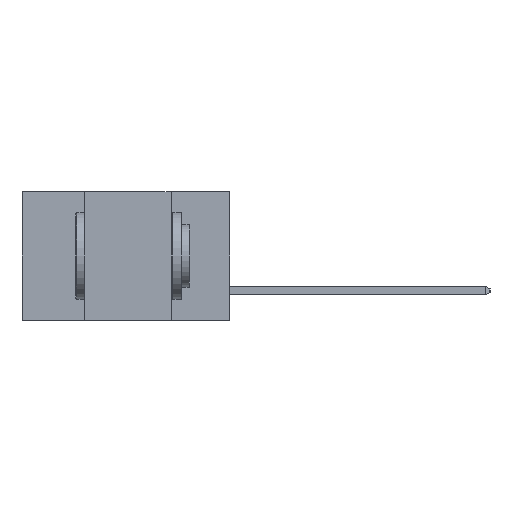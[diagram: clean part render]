
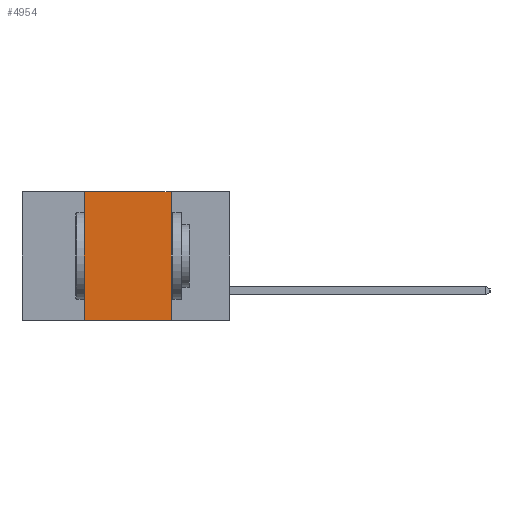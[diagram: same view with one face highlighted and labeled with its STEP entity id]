
A CAD part, left-side view. The second image highlights one B-rep face of the part: STEP entity #4954.
In plain terms, the highlighted planar face has unit normal (-1, 0, 0).
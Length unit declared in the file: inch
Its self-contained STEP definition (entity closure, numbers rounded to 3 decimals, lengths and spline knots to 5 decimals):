
#1108 = LINE ( 'NONE', #4610, #4669 ) ;
#2215 = LINE ( 'NONE', #11364, #16387 ) ;
#2260 = CARTESIAN_POINT ( 'NONE',  ( 0., 0.6, -0.37 ) ) ;
#2921 = CARTESIAN_POINT ( 'NONE',  ( 0., 0.42, 0. ) ) ;
#3185 = EDGE_CURVE ( 'NONE', #5543, #7840, #6414, .T. ) ;
#4086 = EDGE_CURVE ( 'NONE', #5543, #10843, #2215, .T. ) ;
#4257 = CARTESIAN_POINT ( 'NONE',  ( 0., 0.42, -0.37 ) ) ;
#4472 = DIRECTION ( 'NONE',  ( 0., 0., -1. ) ) ;
#4539 = ORIENTED_EDGE ( 'NONE', *, *, #4086, .F. ) ;
#4610 = CARTESIAN_POINT ( 'NONE',  ( 0., 0.6, 0. ) ) ;
#4669 = VECTOR ( 'NONE', #15276, 39.37008 ) ;
#4676 = PLANE ( 'NONE',  #4802 ) ;
#4802 = AXIS2_PLACEMENT_3D ( 'NONE', #4924, #5004, #4990 ) ;
#4924 = CARTESIAN_POINT ( 'NONE',  ( 0., 0.6, 0. ) ) ;
#4954 = ADVANCED_FACE ( 'NONE', ( #9652 ), #4676, .F. ) ;
#4990 = DIRECTION ( 'NONE',  ( 0., 0., -1. ) ) ;
#5001 = EDGE_CURVE ( 'NONE', #10489, #7840, #15945, .T. ) ;
#5004 = DIRECTION ( 'NONE',  ( 1., 0., 0. ) ) ;
#5256 = ORIENTED_EDGE ( 'NONE', *, *, #3185, .T. ) ;
#5543 = VERTEX_POINT ( 'NONE', #4257 ) ;
#5583 = CARTESIAN_POINT ( 'NONE',  ( 0., 0.17, 0. ) ) ;
#5687 = EDGE_CURVE ( 'NONE', #10843, #10489, #1108, .T. ) ;
#5788 = ORIENTED_EDGE ( 'NONE', *, *, #5001, .F. ) ;
#6007 = ORIENTED_EDGE ( 'NONE', *, *, #5687, .F. ) ;
#6414 = LINE ( 'NONE', #2260, #9906 ) ;
#7691 = CARTESIAN_POINT ( 'NONE',  ( 0., 0.17, -0.37 ) ) ;
#7840 = VERTEX_POINT ( 'NONE', #7691 ) ;
#8431 = VECTOR ( 'NONE', #4472, 39.37008 ) ;
#9652 = FACE_OUTER_BOUND ( 'NONE', #11550, .T. ) ;
#9906 = VECTOR ( 'NONE', #12472, 39.37008 ) ;
#10134 = CARTESIAN_POINT ( 'NONE',  ( 0., 0.17, 0. ) ) ;
#10489 = VERTEX_POINT ( 'NONE', #10134 ) ;
#10843 = VERTEX_POINT ( 'NONE', #2921 ) ;
#11364 = CARTESIAN_POINT ( 'NONE',  ( 0., 0.42, 0. ) ) ;
#11383 = DIRECTION ( 'NONE',  ( 0., 0., 1. ) ) ;
#11550 = EDGE_LOOP ( 'NONE', ( #5788, #6007, #4539, #5256 ) ) ;
#12472 = DIRECTION ( 'NONE',  ( 0., -1., 0. ) ) ;
#15276 = DIRECTION ( 'NONE',  ( 0., -1., 0. ) ) ;
#15945 = LINE ( 'NONE', #5583, #8431 ) ;
#16387 = VECTOR ( 'NONE', #11383, 39.37008 ) ;
